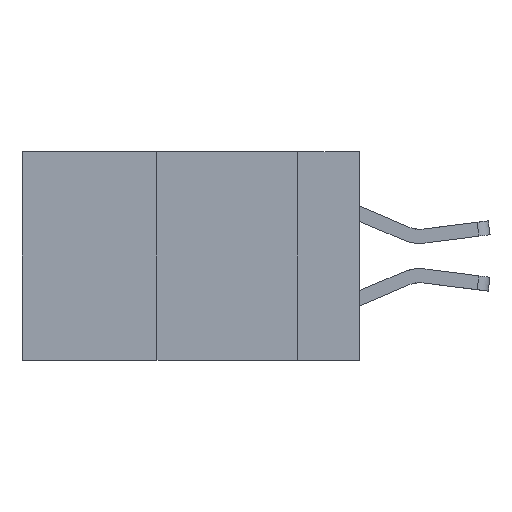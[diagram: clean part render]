
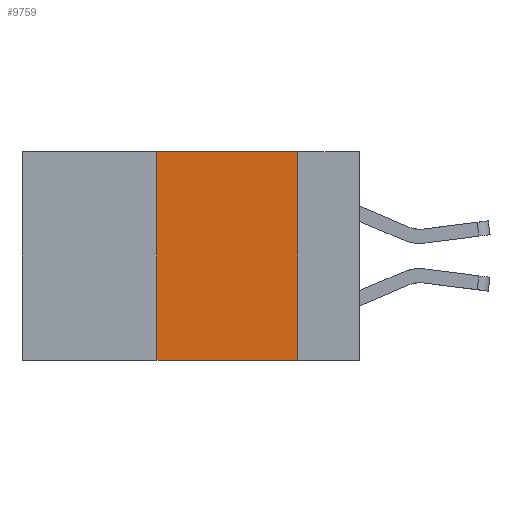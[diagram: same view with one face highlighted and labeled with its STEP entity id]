
A CAD part, left-side view. The second image highlights one B-rep face of the part: STEP entity #9759.
In plain terms, the highlighted planar face has unit normal (-1, 0, 0).
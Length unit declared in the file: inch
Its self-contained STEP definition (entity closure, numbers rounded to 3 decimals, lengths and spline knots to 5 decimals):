
#727 = CARTESIAN_POINT ( 'NONE',  ( 0., 0.6, 0. ) ) ;
#1254 = CARTESIAN_POINT ( 'NONE',  ( 0., 0.36, 0. ) ) ;
#1500 = VERTEX_POINT ( 'NONE', #9630 ) ;
#1876 = DIRECTION ( 'NONE',  ( 0., -1., 0. ) ) ;
#3246 = VECTOR ( 'NONE', #4749, 39.37008 ) ;
#3408 = CARTESIAN_POINT ( 'NONE',  ( 0., 0.11, 0. ) ) ;
#3990 = DIRECTION ( 'NONE',  ( 1., 0., 0. ) ) ;
#4749 = DIRECTION ( 'NONE',  ( 0., 0., 1. ) ) ;
#5560 = EDGE_CURVE ( 'NONE', #5687, #13355, #9380, .T. ) ;
#5687 = VERTEX_POINT ( 'NONE', #12851 ) ;
#6152 = EDGE_CURVE ( 'NONE', #6797, #1500, #12824, .T. ) ;
#6574 = ORIENTED_EDGE ( 'NONE', *, *, #10624, .T. ) ;
#6797 = VERTEX_POINT ( 'NONE', #13682 ) ;
#7459 = PLANE ( 'NONE',  #8398 ) ;
#8063 = LINE ( 'NONE', #727, #13504 ) ;
#8398 = AXIS2_PLACEMENT_3D ( 'NONE', #10853, #3990, #12034 ) ;
#8989 = VECTOR ( 'NONE', #14431, 39.37008 ) ;
#9380 = LINE ( 'NONE', #1254, #3246 ) ;
#9630 = CARTESIAN_POINT ( 'NONE',  ( 0., 0.11, -0.37 ) ) ;
#9707 = LINE ( 'NONE', #11330, #8989 ) ;
#9759 = ADVANCED_FACE ( 'NONE', ( #9890 ), #7459, .F. ) ;
#9885 = VECTOR ( 'NONE', #11511, 39.37008 ) ;
#9890 = FACE_OUTER_BOUND ( 'NONE', #10730, .T. ) ;
#10138 = ORIENTED_EDGE ( 'NONE', *, *, #5560, .F. ) ;
#10624 = EDGE_CURVE ( 'NONE', #5687, #1500, #9707, .T. ) ;
#10663 = ORIENTED_EDGE ( 'NONE', *, *, #6152, .F. ) ;
#10730 = EDGE_LOOP ( 'NONE', ( #10663, #11969, #10138, #6574 ) ) ;
#10853 = CARTESIAN_POINT ( 'NONE',  ( 0., 0.6, 0. ) ) ;
#11330 = CARTESIAN_POINT ( 'NONE',  ( 0., 0.6, -0.37 ) ) ;
#11511 = DIRECTION ( 'NONE',  ( 0., 0., -1. ) ) ;
#11969 = ORIENTED_EDGE ( 'NONE', *, *, #14389, .F. ) ;
#12034 = DIRECTION ( 'NONE',  ( 0., 0., -1. ) ) ;
#12345 = CARTESIAN_POINT ( 'NONE',  ( 0., 0.36, 0. ) ) ;
#12824 = LINE ( 'NONE', #3408, #9885 ) ;
#12851 = CARTESIAN_POINT ( 'NONE',  ( 0., 0.36, -0.37 ) ) ;
#13355 = VERTEX_POINT ( 'NONE', #12345 ) ;
#13504 = VECTOR ( 'NONE', #1876, 39.37008 ) ;
#13682 = CARTESIAN_POINT ( 'NONE',  ( 0., 0.11, 0. ) ) ;
#14389 = EDGE_CURVE ( 'NONE', #13355, #6797, #8063, .T. ) ;
#14431 = DIRECTION ( 'NONE',  ( 0., -1., 0. ) ) ;
